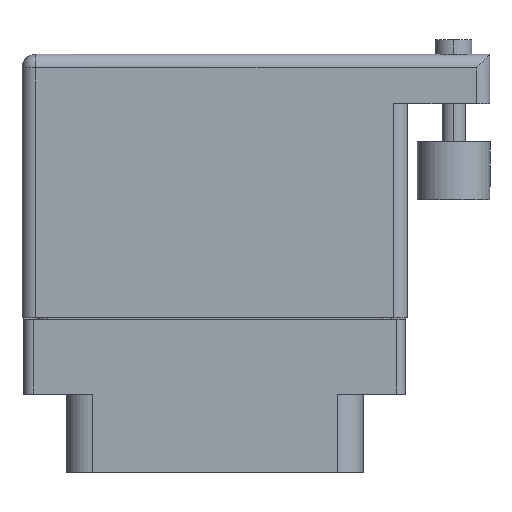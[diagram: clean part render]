
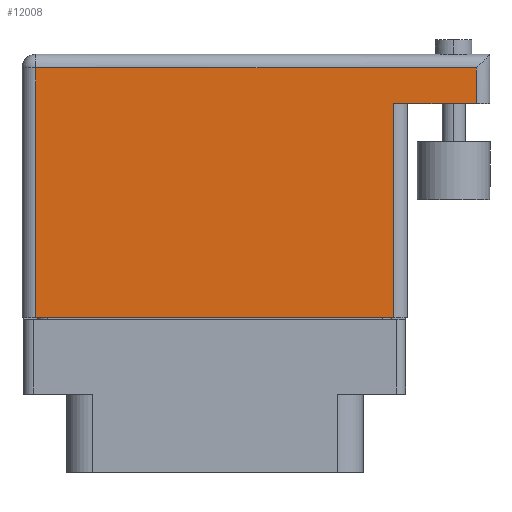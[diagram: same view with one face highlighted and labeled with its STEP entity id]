
A CAD part, front view. The second image highlights one B-rep face of the part: STEP entity #12008.
In plain terms, the highlighted face is planar.
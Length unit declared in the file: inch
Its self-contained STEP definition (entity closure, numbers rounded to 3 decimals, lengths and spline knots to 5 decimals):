
#130 = DIRECTION ( 'NONE',  ( -1., 0., 0. ) ) ;
#298 = PLANE ( 'NONE',  #22371 ) ;
#639 = CARTESIAN_POINT ( 'NONE',  ( -0.6155, -0.1, 0.3575 ) ) ;
#2044 = EDGE_CURVE ( 'NONE', #18991, #22050, #20422, .T. ) ;
#4215 = VERTEX_POINT ( 'NONE', #7356 ) ;
#4332 = DIRECTION ( 'NONE',  ( 0., 1., 0. ) ) ;
#4370 = ORIENTED_EDGE ( 'NONE', *, *, #21606, .T. ) ;
#4563 = LINE ( 'NONE', #12556, #19489 ) ;
#5187 = VECTOR ( 'NONE', #7987, 39.37008 ) ;
#5947 = DIRECTION ( 'NONE',  ( 0., 0., -1. ) ) ;
#6383 = VECTOR ( 'NONE', #10639, 39.37008 ) ;
#6418 = FACE_OUTER_BOUND ( 'NONE', #21455, .T. ) ;
#6541 = CARTESIAN_POINT ( 'NONE',  ( 0.8995, 0.759, 0.3575 ) ) ;
#6659 = CARTESIAN_POINT ( 'NONE',  ( 0.6155, 0.636, 0.3575 ) ) ;
#7356 = CARTESIAN_POINT ( 'NONE',  ( -0.6155, 0.759, 0.3575 ) ) ;
#7725 = CARTESIAN_POINT ( 'NONE',  ( -0.6625, -0.1, 0.3575 ) ) ;
#7797 = CARTESIAN_POINT ( 'NONE',  ( 0.8995, 0.636, 0.3575 ) ) ;
#7987 = DIRECTION ( 'NONE',  ( 1., 0., 0. ) ) ;
#8017 = ORIENTED_EDGE ( 'NONE', *, *, #16473, .T. ) ;
#8718 = VECTOR ( 'NONE', #22116, 39.37008 ) ;
#9392 = CARTESIAN_POINT ( 'NONE',  ( 0.6155, 0.636, 0.3575 ) ) ;
#9850 = CARTESIAN_POINT ( 'NONE',  ( -0.6155, -0.1, 0.3575 ) ) ;
#10250 = CARTESIAN_POINT ( 'NONE',  ( 0.9465, 0.636, 0.3575 ) ) ;
#10639 = DIRECTION ( 'NONE',  ( 0., -1., 0. ) ) ;
#12008 = ADVANCED_FACE ( 'NONE', ( #6418 ), #298, .F. ) ;
#12312 = VERTEX_POINT ( 'NONE', #9392 ) ;
#12556 = CARTESIAN_POINT ( 'NONE',  ( 0.8995, 0.806, 0.3575 ) ) ;
#12728 = DIRECTION ( 'NONE',  ( 0., 1., 0. ) ) ;
#12733 = ORIENTED_EDGE ( 'NONE', *, *, #17934, .F. ) ;
#14416 = LINE ( 'NONE', #19968, #8718 ) ;
#14428 = DIRECTION ( 'NONE',  ( -1., 0., 0. ) ) ;
#15201 = VECTOR ( 'NONE', #14428, 39.37008 ) ;
#16473 = EDGE_CURVE ( 'NONE', #17164, #4215, #14416, .T. ) ;
#16493 = VERTEX_POINT ( 'NONE', #7797 ) ;
#16568 = ORIENTED_EDGE ( 'NONE', *, *, #17507, .T. ) ;
#16874 = ORIENTED_EDGE ( 'NONE', *, *, #22768, .T. ) ;
#17164 = VERTEX_POINT ( 'NONE', #6541 ) ;
#17507 = EDGE_CURVE ( 'NONE', #22050, #12312, #26212, .T. ) ;
#17934 = EDGE_CURVE ( 'NONE', #16493, #12312, #24787, .T. ) ;
#18991 = VERTEX_POINT ( 'NONE', #9850 ) ;
#19489 = VECTOR ( 'NONE', #12728, 39.37008 ) ;
#19968 = CARTESIAN_POINT ( 'NONE',  ( -0.6625, 0.759, 0.3575 ) ) ;
#20319 = CARTESIAN_POINT ( 'NONE',  ( -0.6625, 0.806, 0.3575 ) ) ;
#20357 = LINE ( 'NONE', #639, #6383 ) ;
#20422 = LINE ( 'NONE', #7725, #5187 ) ;
#21247 = ORIENTED_EDGE ( 'NONE', *, *, #2044, .T. ) ;
#21455 = EDGE_LOOP ( 'NONE', ( #21247, #16568, #12733, #4370, #8017, #16874 ) ) ;
#21606 = EDGE_CURVE ( 'NONE', #16493, #17164, #4563, .T. ) ;
#22050 = VERTEX_POINT ( 'NONE', #25135 ) ;
#22116 = DIRECTION ( 'NONE',  ( -1., 0., 0. ) ) ;
#22371 = AXIS2_PLACEMENT_3D ( 'NONE', #20319, #5947, #130 ) ;
#22768 = EDGE_CURVE ( 'NONE', #4215, #18991, #20357, .T. ) ;
#22985 = VECTOR ( 'NONE', #4332, 39.37008 ) ;
#24787 = LINE ( 'NONE', #10250, #15201 ) ;
#25135 = CARTESIAN_POINT ( 'NONE',  ( 0.6155, -0.1, 0.3575 ) ) ;
#26212 = LINE ( 'NONE', #6659, #22985 ) ;
